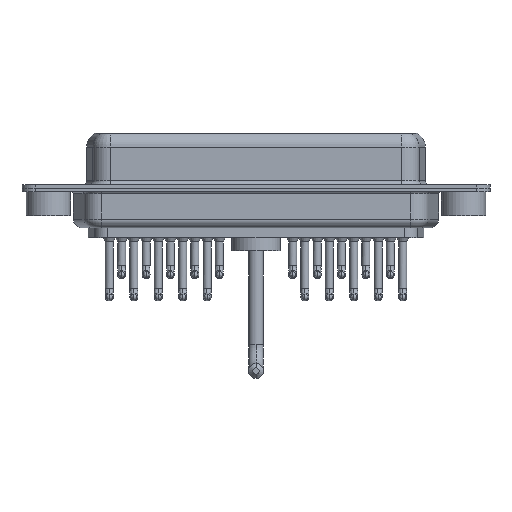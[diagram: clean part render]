
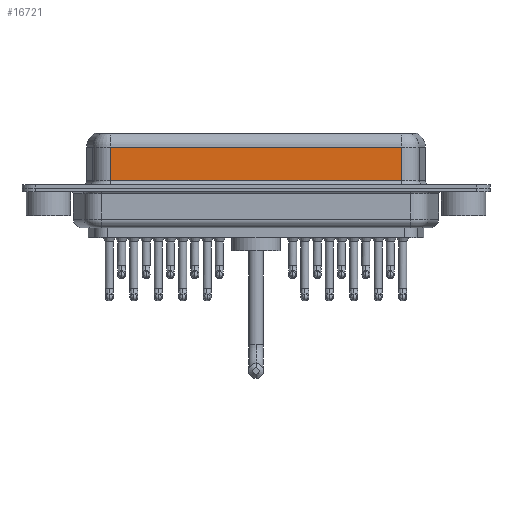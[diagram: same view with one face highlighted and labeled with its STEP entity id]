
A CAD part, front view. The second image highlights one B-rep face of the part: STEP entity #16721.
In plain terms, the highlighted planar face has unit normal (0, -1, 0).
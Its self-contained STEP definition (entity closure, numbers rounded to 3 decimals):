
#204 = EDGE_CURVE ( 'NONE', #17414, #3185, #4219, .T. ) ;
#1097 = CARTESIAN_POINT ( 'NONE',  ( 40.037, -3.95, 6.4 ) ) ;
#1347 = DIRECTION ( 'NONE',  ( 0., 1., 0. ) ) ;
#1664 = CARTESIAN_POINT ( 'NONE',  ( 7.013, -3.95, 0.9 ) ) ;
#3021 = EDGE_CURVE ( 'NONE', #19883, #3185, #13070, .T. ) ;
#3157 = ORIENTED_EDGE ( 'NONE', *, *, #3021, .F. ) ;
#3185 = VERTEX_POINT ( 'NONE', #21062 ) ;
#3605 = EDGE_CURVE ( 'NONE', #19883, #14738, #19907, .T. ) ;
#4219 = LINE ( 'NONE', #5710, #15967 ) ;
#4732 = VECTOR ( 'NONE', #14986, 1000. ) ;
#5710 = CARTESIAN_POINT ( 'NONE',  ( 40.037, -3.95, 0.9 ) ) ;
#6061 = DIRECTION ( 'NONE',  ( 0., 0., -1. ) ) ;
#8576 = ORIENTED_EDGE ( 'NONE', *, *, #11166, .T. ) ;
#9927 = CARTESIAN_POINT ( 'NONE',  ( 40.037, -3.95, 4.65 ) ) ;
#10197 = DIRECTION ( 'NONE',  ( 0., 0., 1. ) ) ;
#10291 = AXIS2_PLACEMENT_3D ( 'NONE', #22356, #1347, #10197 ) ;
#10634 = VECTOR ( 'NONE', #6061, 1000. ) ;
#11166 = EDGE_CURVE ( 'NONE', #14738, #17414, #18208, .T. ) ;
#12731 = DIRECTION ( 'NONE',  ( 1., 0., 0. ) ) ;
#12815 = VECTOR ( 'NONE', #19813, 1000. ) ;
#13070 = LINE ( 'NONE', #1097, #10634 ) ;
#14738 = VERTEX_POINT ( 'NONE', #22176 ) ;
#14986 = DIRECTION ( 'NONE',  ( -1., 0., 0. ) ) ;
#15257 = FACE_OUTER_BOUND ( 'NONE', #19811, .T. ) ;
#15964 = ORIENTED_EDGE ( 'NONE', *, *, #204, .T. ) ;
#15967 = VECTOR ( 'NONE', #12731, 1000. ) ;
#16721 = ADVANCED_FACE ( 'NONE', ( #15257 ), #16758, .F. ) ;
#16758 = PLANE ( 'NONE',  #10291 ) ;
#17414 = VERTEX_POINT ( 'NONE', #1664 ) ;
#18208 = LINE ( 'NONE', #21324, #12815 ) ;
#19811 = EDGE_LOOP ( 'NONE', ( #3157, #22613, #8576, #15964 ) ) ;
#19813 = DIRECTION ( 'NONE',  ( 0., 0., -1. ) ) ;
#19883 = VERTEX_POINT ( 'NONE', #20089 ) ;
#19907 = LINE ( 'NONE', #9927, #4732 ) ;
#20089 = CARTESIAN_POINT ( 'NONE',  ( 40.037, -3.95, 4.65 ) ) ;
#21062 = CARTESIAN_POINT ( 'NONE',  ( 40.037, -3.95, 0.9 ) ) ;
#21324 = CARTESIAN_POINT ( 'NONE',  ( 7.013, -3.95, 6.4 ) ) ;
#22176 = CARTESIAN_POINT ( 'NONE',  ( 7.013, -3.95, 4.65 ) ) ;
#22356 = CARTESIAN_POINT ( 'NONE',  ( 40.037, -3.95, 6.4 ) ) ;
#22613 = ORIENTED_EDGE ( 'NONE', *, *, #3605, .T. ) ;
